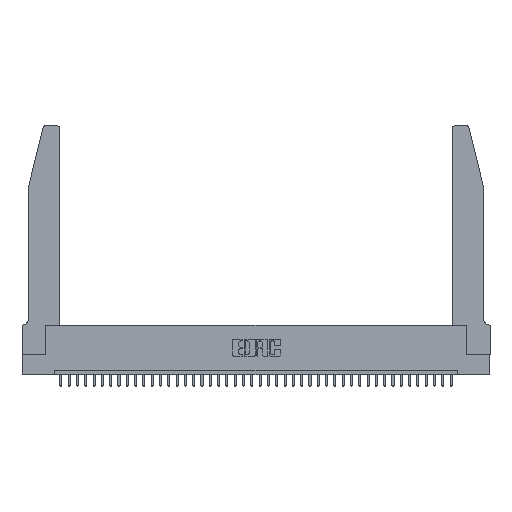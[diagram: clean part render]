
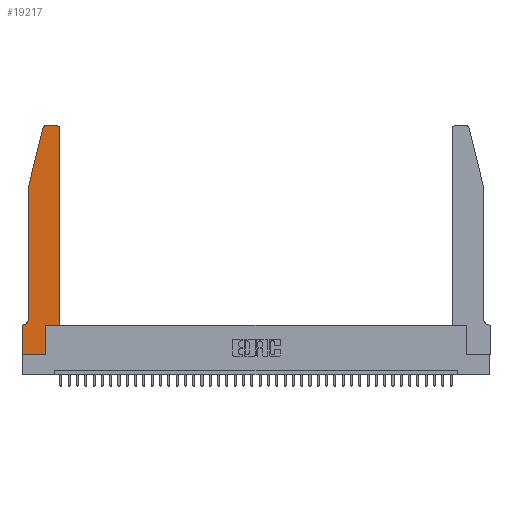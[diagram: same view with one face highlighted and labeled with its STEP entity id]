
A CAD part, top view. The second image highlights one B-rep face of the part: STEP entity #19217.
In plain terms, the highlighted planar face has unit normal (0, 0, 1).
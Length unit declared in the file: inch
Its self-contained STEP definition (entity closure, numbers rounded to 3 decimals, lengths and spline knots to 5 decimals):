
#213 = CARTESIAN_POINT ( 'NONE',  ( 0.25487, 2.72718, 0.37 ) ) ;
#434 = CARTESIAN_POINT ( 'NONE',  ( 0.2605, 2.75, 0.37 ) ) ;
#841 = DIRECTION ( 'NONE',  ( 1., 0., 0. ) ) ;
#1110 = EDGE_CURVE ( 'NONE', #27606, #38982, #33192, .T. ) ;
#2077 = DIRECTION ( 'NONE',  ( -0.239, -0.971, 0. ) ) ;
#2389 = EDGE_LOOP ( 'NONE', ( #32401, #34504, #13104, #28315, #22338, #18556, #34844, #17039, #33799, #26570, #31114, #18627 ) ) ;
#3019 = DIRECTION ( 'NONE',  ( 1., 0., 0. ) ) ;
#3733 = DIRECTION ( 'NONE',  ( 0., -1., 0. ) ) ;
#4526 = DIRECTION ( 'NONE',  ( 0., 0., -1. ) ) ;
#5723 = FACE_OUTER_BOUND ( 'NONE', #2389, .T. ) ;
#5957 = CARTESIAN_POINT ( 'NONE',  ( 0., 0.35, 0.37 ) ) ;
#6245 = VERTEX_POINT ( 'NONE', #213 ) ;
#6658 = EDGE_CURVE ( 'NONE', #11586, #20944, #38141, .T. ) ;
#6827 = LINE ( 'NONE', #10085, #8793 ) ;
#6942 = DIRECTION ( 'NONE',  ( 0., 0., 1. ) ) ;
#7127 = LINE ( 'NONE', #35230, #33259 ) ;
#7386 = DIRECTION ( 'NONE',  ( -1., 0., 0. ) ) ;
#7547 = CARTESIAN_POINT ( 'NONE',  ( 0.0755, 0.42, 0.37 ) ) ;
#7865 = AXIS2_PLACEMENT_3D ( 'NONE', #21378, #34210, #3019 ) ;
#8793 = VECTOR ( 'NONE', #19515, 39.37008 ) ;
#9240 = DIRECTION ( 'NONE',  ( 0., 0., 1. ) ) ;
#9437 = LINE ( 'NONE', #19424, #33111 ) ;
#10085 = CARTESIAN_POINT ( 'NONE',  ( 0., 0., 0.37 ) ) ;
#10779 = VECTOR ( 'NONE', #2077, 39.37008 ) ;
#11288 = CARTESIAN_POINT ( 'NONE',  ( 0.2865, 0.35, 0.37 ) ) ;
#11294 = VECTOR ( 'NONE', #37711, 39.37008 ) ;
#11586 = VERTEX_POINT ( 'NONE', #29241 ) ;
#11847 = CARTESIAN_POINT ( 'NONE',  ( 0.4505, 0.35, 0.37 ) ) ;
#12067 = EDGE_CURVE ( 'NONE', #13380, #29911, #15277, .T. ) ;
#12706 = LINE ( 'NONE', #14661, #10779 ) ;
#13104 = ORIENTED_EDGE ( 'NONE', *, *, #23926, .T. ) ;
#13223 = VERTEX_POINT ( 'NONE', #37379 ) ;
#13380 = VERTEX_POINT ( 'NONE', #26601 ) ;
#13471 = CARTESIAN_POINT ( 'NONE',  ( 0.4205, 2.72, 0.37 ) ) ;
#13777 = CARTESIAN_POINT ( 'NONE',  ( 0.4205, 2.75, 0.37 ) ) ;
#14661 = CARTESIAN_POINT ( 'NONE',  ( 0.0755, 2., 0.37 ) ) ;
#15277 = LINE ( 'NONE', #15971, #28313 ) ;
#15285 = EDGE_CURVE ( 'NONE', #20944, #27606, #34923, .T. ) ;
#15938 = CARTESIAN_POINT ( 'NONE',  ( 0.0055, 0.35, 0.37 ) ) ;
#15971 = CARTESIAN_POINT ( 'NONE',  ( 0., 0., 0.37 ) ) ;
#16748 = DIRECTION ( 'NONE',  ( -1., 0., 0. ) ) ;
#17039 = ORIENTED_EDGE ( 'NONE', *, *, #37552, .T. ) ;
#18235 = DIRECTION ( 'NONE',  ( 1., 0., 0. ) ) ;
#18545 = DIRECTION ( 'NONE',  ( 0., -1., 0. ) ) ;
#18556 = ORIENTED_EDGE ( 'NONE', *, *, #31753, .T. ) ;
#18627 = ORIENTED_EDGE ( 'NONE', *, *, #1110, .T. ) ;
#19217 = ADVANCED_FACE ( 'NONE', ( #5723 ), #24483, .T. ) ;
#19424 = CARTESIAN_POINT ( 'NONE',  ( 0.0755, 2., 0.37 ) ) ;
#19515 = DIRECTION ( 'NONE',  ( 1., 0., 0. ) ) ;
#20257 = VECTOR ( 'NONE', #18235, 39.37008 ) ;
#20944 = VERTEX_POINT ( 'NONE', #11847 ) ;
#21180 = CARTESIAN_POINT ( 'NONE',  ( 0.4505, 0.35, 0.37 ) ) ;
#21378 = CARTESIAN_POINT ( 'NONE',  ( 0.284, 2.72, 0.37 ) ) ;
#22299 = CARTESIAN_POINT ( 'NONE',  ( 0.4505, 2.72, 0.37 ) ) ;
#22338 = ORIENTED_EDGE ( 'NONE', *, *, #25707, .T. ) ;
#22350 = VECTOR ( 'NONE', #27769, 39.37008 ) ;
#23066 = EDGE_CURVE ( 'NONE', #38982, #38448, #31545, .T. ) ;
#23661 = DIRECTION ( 'NONE',  ( 0., 1., 0. ) ) ;
#23708 = VERTEX_POINT ( 'NONE', #24019 ) ;
#23770 = CIRCLE ( 'NONE', #7865, 0.03 ) ;
#23926 = EDGE_CURVE ( 'NONE', #6245, #23708, #12706, .T. ) ;
#24019 = CARTESIAN_POINT ( 'NONE',  ( 0.0755, 2., 0.37 ) ) ;
#24063 = VERTEX_POINT ( 'NONE', #15938 ) ;
#24483 = PLANE ( 'NONE',  #31786 ) ;
#24493 = CARTESIAN_POINT ( 'NONE',  ( 0.4505, 0.35, 0.37 ) ) ;
#24494 = VECTOR ( 'NONE', #23661, 39.37008 ) ;
#25707 = EDGE_CURVE ( 'NONE', #37001, #24063, #39675, .T. ) ;
#26231 = CARTESIAN_POINT ( 'NONE',  ( 0., 0., 0.37 ) ) ;
#26570 = ORIENTED_EDGE ( 'NONE', *, *, #6658, .T. ) ;
#26601 = CARTESIAN_POINT ( 'NONE',  ( 0., 0.35, 0.37 ) ) ;
#27606 = VERTEX_POINT ( 'NONE', #22299 ) ;
#27768 = EDGE_CURVE ( 'NONE', #13223, #11586, #32709, .T. ) ;
#27769 = DIRECTION ( 'NONE',  ( -1., 0., 0. ) ) ;
#28313 = VECTOR ( 'NONE', #18545, 39.37008 ) ;
#28315 = ORIENTED_EDGE ( 'NONE', *, *, #29167, .T. ) ;
#29167 = EDGE_CURVE ( 'NONE', #23708, #37001, #9437, .T. ) ;
#29241 = CARTESIAN_POINT ( 'NONE',  ( 0.2865, 0.35, 0.37 ) ) ;
#29911 = VERTEX_POINT ( 'NONE', #26231 ) ;
#30823 = DIRECTION ( 'NONE',  ( 1., 0., 0. ) ) ;
#30874 = EDGE_CURVE ( 'NONE', #38448, #6245, #23770, .T. ) ;
#31114 = ORIENTED_EDGE ( 'NONE', *, *, #15285, .T. ) ;
#31545 = LINE ( 'NONE', #434, #22350 ) ;
#31753 = EDGE_CURVE ( 'NONE', #24063, #13380, #7127, .T. ) ;
#31786 = AXIS2_PLACEMENT_3D ( 'NONE', #5957, #9240, #30823 ) ;
#32401 = ORIENTED_EDGE ( 'NONE', *, *, #23066, .T. ) ;
#32709 = LINE ( 'NONE', #11288, #24494 ) ;
#32958 = CARTESIAN_POINT ( 'NONE',  ( 0.284, 2.75, 0.37 ) ) ;
#33111 = VECTOR ( 'NONE', #3733, 39.37008 ) ;
#33192 = CIRCLE ( 'NONE', #34534, 0.03 ) ;
#33259 = VECTOR ( 'NONE', #16748, 39.37008 ) ;
#33799 = ORIENTED_EDGE ( 'NONE', *, *, #27768, .T. ) ;
#34210 = DIRECTION ( 'NONE',  ( 0., 0., 1. ) ) ;
#34504 = ORIENTED_EDGE ( 'NONE', *, *, #30874, .T. ) ;
#34534 = AXIS2_PLACEMENT_3D ( 'NONE', #13471, #6942, #841 ) ;
#34844 = ORIENTED_EDGE ( 'NONE', *, *, #12067, .T. ) ;
#34923 = LINE ( 'NONE', #24493, #11294 ) ;
#35201 = AXIS2_PLACEMENT_3D ( 'NONE', #38445, #4526, #7386 ) ;
#35230 = CARTESIAN_POINT ( 'NONE',  ( 0.0755, 0.35, 0.37 ) ) ;
#37001 = VERTEX_POINT ( 'NONE', #7547 ) ;
#37379 = CARTESIAN_POINT ( 'NONE',  ( 0.2865, 0., 0.37 ) ) ;
#37552 = EDGE_CURVE ( 'NONE', #29911, #13223, #6827, .T. ) ;
#37711 = DIRECTION ( 'NONE',  ( 0., 1., 0. ) ) ;
#38141 = LINE ( 'NONE', #21180, #20257 ) ;
#38445 = CARTESIAN_POINT ( 'NONE',  ( 0.0055, 0.42, 0.37 ) ) ;
#38448 = VERTEX_POINT ( 'NONE', #32958 ) ;
#38982 = VERTEX_POINT ( 'NONE', #13777 ) ;
#39675 = CIRCLE ( 'NONE', #35201, 0.07 ) ;
